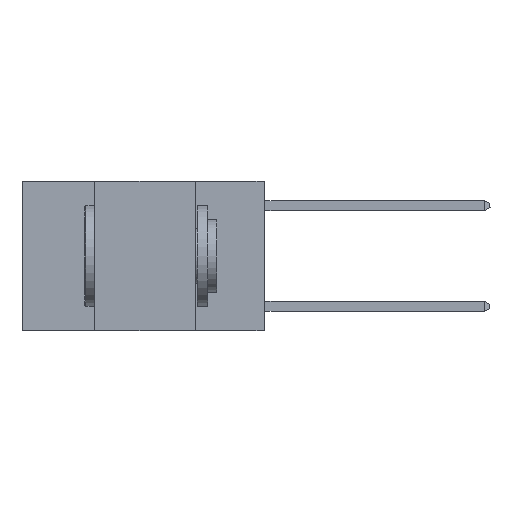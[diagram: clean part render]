
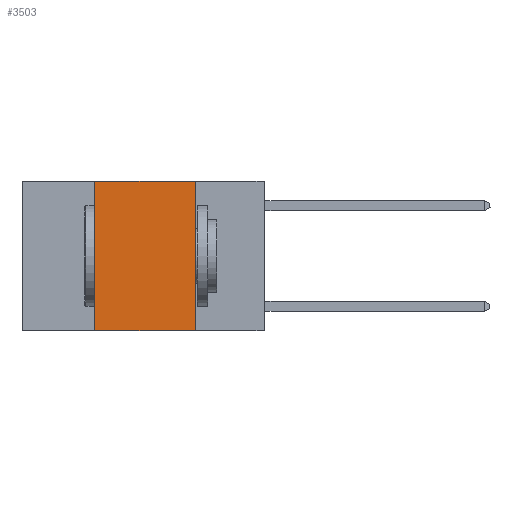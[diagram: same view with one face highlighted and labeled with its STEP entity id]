
A CAD part, left-side view. The second image highlights one B-rep face of the part: STEP entity #3503.
In plain terms, the highlighted planar face has unit normal (-1, 0, 0).
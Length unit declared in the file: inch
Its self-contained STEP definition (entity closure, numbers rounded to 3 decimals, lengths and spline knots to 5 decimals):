
#243 = LINE ( 'NONE', #12435, #9402 ) ;
#354 = LINE ( 'NONE', #9718, #3174 ) ;
#364 = EDGE_CURVE ( 'NONE', #11651, #2249, #243, .T. ) ;
#422 = LINE ( 'NONE', #3578, #8856 ) ;
#553 = CARTESIAN_POINT ( 'NONE',  ( 0., 0.42, 0. ) ) ;
#584 = VECTOR ( 'NONE', #4026, 39.37008 ) ;
#728 = CARTESIAN_POINT ( 'NONE',  ( 0., 0.6, 0. ) ) ;
#1365 = DIRECTION ( 'NONE',  ( 0., 0., -1. ) ) ;
#1713 = VERTEX_POINT ( 'NONE', #553 ) ;
#2249 = VERTEX_POINT ( 'NONE', #9937 ) ;
#2821 = CARTESIAN_POINT ( 'NONE',  ( 0., 0.42, 0. ) ) ;
#3123 = FACE_OUTER_BOUND ( 'NONE', #5012, .T. ) ;
#3174 = VECTOR ( 'NONE', #1365, 39.37008 ) ;
#3503 = ADVANCED_FACE ( 'NONE', ( #3123 ), #12643, .F. ) ;
#3578 = CARTESIAN_POINT ( 'NONE',  ( 0., 0.6, 0. ) ) ;
#3771 = LINE ( 'NONE', #2821, #584 ) ;
#4026 = DIRECTION ( 'NONE',  ( 0., 0., 1. ) ) ;
#5012 = EDGE_LOOP ( 'NONE', ( #15000, #7513, #8888, #8447 ) ) ;
#5026 = VERTEX_POINT ( 'NONE', #11880 ) ;
#6298 = EDGE_CURVE ( 'NONE', #11651, #1713, #3771, .T. ) ;
#6759 = DIRECTION ( 'NONE',  ( 0., 0., -1. ) ) ;
#7303 = EDGE_CURVE ( 'NONE', #5026, #2249, #354, .T. ) ;
#7513 = ORIENTED_EDGE ( 'NONE', *, *, #10988, .F. ) ;
#8447 = ORIENTED_EDGE ( 'NONE', *, *, #364, .T. ) ;
#8856 = VECTOR ( 'NONE', #9509, 39.37008 ) ;
#8888 = ORIENTED_EDGE ( 'NONE', *, *, #6298, .F. ) ;
#9402 = VECTOR ( 'NONE', #10191, 39.37008 ) ;
#9509 = DIRECTION ( 'NONE',  ( 0., -1., 0. ) ) ;
#9718 = CARTESIAN_POINT ( 'NONE',  ( 0., 0.17, 0. ) ) ;
#9937 = CARTESIAN_POINT ( 'NONE',  ( 0., 0.17, -0.37 ) ) ;
#10191 = DIRECTION ( 'NONE',  ( 0., -1., 0. ) ) ;
#10712 = CARTESIAN_POINT ( 'NONE',  ( 0., 0.42, -0.37 ) ) ;
#10988 = EDGE_CURVE ( 'NONE', #1713, #5026, #422, .T. ) ;
#11651 = VERTEX_POINT ( 'NONE', #10712 ) ;
#11880 = CARTESIAN_POINT ( 'NONE',  ( 0., 0.17, 0. ) ) ;
#12435 = CARTESIAN_POINT ( 'NONE',  ( 0., 0.6, -0.37 ) ) ;
#12643 = PLANE ( 'NONE',  #13800 ) ;
#13756 = DIRECTION ( 'NONE',  ( 1., 0., 0. ) ) ;
#13800 = AXIS2_PLACEMENT_3D ( 'NONE', #728, #13756, #6759 ) ;
#15000 = ORIENTED_EDGE ( 'NONE', *, *, #7303, .F. ) ;
